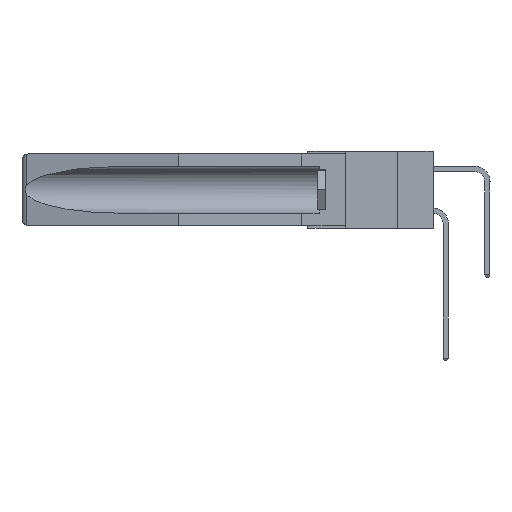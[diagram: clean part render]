
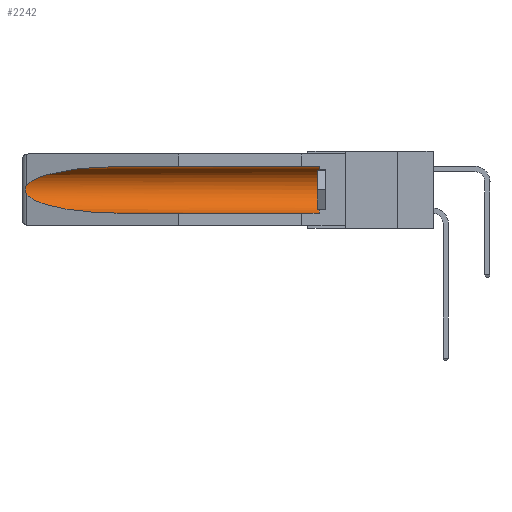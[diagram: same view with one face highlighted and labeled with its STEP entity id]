
A CAD part, left-side view. The second image highlights one B-rep face of the part: STEP entity #2242.
In plain terms, the highlighted cylindrical face has radius 2.857 mm (diameter 5.715 mm), a partial arc.
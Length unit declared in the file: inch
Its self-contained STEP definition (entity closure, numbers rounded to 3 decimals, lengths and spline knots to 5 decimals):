
#13 = VERTEX_POINT ( 'NONE', #9260 ) ;
#589 = ORIENTED_EDGE ( 'NONE', *, *, #10933, .T. ) ;
#742 = CARTESIAN_POINT ( 'NONE',  ( 0.155, 1.07973, -0.059 ) ) ;
#765 = ORIENTED_EDGE ( 'NONE', *, *, #4524, .T. ) ;
#1241 = EDGE_LOOP ( 'NONE', ( #765, #589, #7309, #15230, #18197, #17790 ) ) ;
#1487 = CARTESIAN_POINT ( 'NONE',  ( 0.2675, 1.53308, -0.16763 ) ) ;
#2242 = ADVANCED_FACE ( 'NONE', ( #5202 ), #18464, .F. ) ;
#2340 = DIRECTION ( 'NONE',  ( 0., 0., 1. ) ) ;
#2880 = EDGE_CURVE ( 'NONE', #13, #15522, #5535, .T. ) ;
#3206 = CARTESIAN_POINT ( 'NONE',  ( 0.155, -0.30754, -0.1715 ) ) ;
#3468 = CARTESIAN_POINT ( 'NONE',  ( 0.26537, 1.52718, -0.14972 ) ) ;
#3616 =( BOUNDED_CURVE ( )  B_SPLINE_CURVE ( 3, ( #16390, #7421, #14693, #18410 ),
 .UNSPECIFIED., .F., .F. ) 
 B_SPLINE_CURVE_WITH_KNOTS ( ( 4, 4 ),
 ( 0.1948, 1.5708 ),
 .UNSPECIFIED. ) 
 CURVE ( )  GEOMETRIC_REPRESENTATION_ITEM ( )  RATIONAL_B_SPLINE_CURVE ( ( 1., 0.848, 0.848, 1. ) ) 
 REPRESENTATION_ITEM ( '' )  );
#3846 = EDGE_CURVE ( 'NONE', #11612, #7473, #5758, .T. ) ;
#4273 = DIRECTION ( 'NONE',  ( 0., 1., 0. ) ) ;
#4432 = CARTESIAN_POINT ( 'NONE',  ( 0.155, -0.30754, -0.059 ) ) ;
#4524 = EDGE_CURVE ( 'NONE', #15522, #22439, #20083, .T. ) ;
#5050 = CARTESIAN_POINT ( 'NONE',  ( 0.26597, 1.52961, -0.15275 ) ) ;
#5202 = FACE_OUTER_BOUND ( 'NONE', #1241, .T. ) ;
#5276 = CARTESIAN_POINT ( 'NONE',  ( 0.2675, 1.53308, -0.17534 ) ) ;
#5384 = DIRECTION ( 'NONE',  ( 0., 0., 1. ) ) ;
#5535 = LINE ( 'NONE', #4432, #21639 ) ;
#5715 = CARTESIAN_POINT ( 'NONE',  ( 0.155, -0.30754, -0.284 ) ) ;
#5758 = LINE ( 'NONE', #5715, #20157 ) ;
#7075 = CARTESIAN_POINT ( 'NONE',  ( 0.26537, 1.52718, -0.19328 ) ) ;
#7309 = ORIENTED_EDGE ( 'NONE', *, *, #11479, .T. ) ;
#7373 = CARTESIAN_POINT ( 'NONE',  ( 0.26537, 1.52718, -0.19328 ) ) ;
#7421 = CARTESIAN_POINT ( 'NONE',  ( 0.25451, 1.48313, -0.24835 ) ) ;
#7473 = VERTEX_POINT ( 'NONE', #18750 ) ;
#8163 = EDGE_CURVE ( 'NONE', #11612, #13, #21023, .T. ) ;
#9057 = CARTESIAN_POINT ( 'NONE',  ( 0.25451, 1.48313, -0.09465 ) ) ;
#9208 = CARTESIAN_POINT ( 'NONE',  ( 0.21114, 1.30732, -0.059 ) ) ;
#9260 = CARTESIAN_POINT ( 'NONE',  ( 0.155, 0.126, -0.059 ) ) ;
#9945 = AXIS2_PLACEMENT_3D ( 'NONE', #20248, #14707, #2340 ) ;
#10933 = EDGE_CURVE ( 'NONE', #22439, #11019, #15461, .T. ) ;
#11019 = VERTEX_POINT ( 'NONE', #7373 ) ;
#11479 = EDGE_CURVE ( 'NONE', #11019, #7473, #3616, .T. ) ;
#11612 = VERTEX_POINT ( 'NONE', #22201 ) ;
#14693 = CARTESIAN_POINT ( 'NONE',  ( 0.21114, 1.30732, -0.284 ) ) ;
#14697 = CARTESIAN_POINT ( 'NONE',  ( 0.26537, 1.52718, -0.14972 ) ) ;
#14707 = DIRECTION ( 'NONE',  ( 0., -1., 0. ) ) ;
#15230 = ORIENTED_EDGE ( 'NONE', *, *, #3846, .F. ) ;
#15461 = B_SPLINE_CURVE_WITH_KNOTS ( 'NONE', 3,
 ( #3468, #5050, #16129, #16104, #1487, #5276, #17973, #17895, #19723, #7075 ),
 .UNSPECIFIED., .F., .F.,
 ( 4, 2, 2, 2, 4 ),
 ( 0., 0.00029, 0.00058, 0.00087, 0.00117 ),
 .UNSPECIFIED. ) ;
#15522 = VERTEX_POINT ( 'NONE', #742 ) ;
#16104 = CARTESIAN_POINT ( 'NONE',  ( 0.2673, 1.5327, -0.16383 ) ) ;
#16129 = CARTESIAN_POINT ( 'NONE',  ( 0.26654, 1.53092, -0.15636 ) ) ;
#16315 = DIRECTION ( 'NONE',  ( 0., 1., 0. ) ) ;
#16390 = CARTESIAN_POINT ( 'NONE',  ( 0.26537, 1.52718, -0.19328 ) ) ;
#17627 = CARTESIAN_POINT ( 'NONE',  ( 0.26537, 1.52718, -0.14972 ) ) ;
#17790 = ORIENTED_EDGE ( 'NONE', *, *, #2880, .T. ) ;
#17895 = CARTESIAN_POINT ( 'NONE',  ( 0.26655, 1.53094, -0.18657 ) ) ;
#17973 = CARTESIAN_POINT ( 'NONE',  ( 0.2673, 1.53269, -0.17917 ) ) ;
#18197 = ORIENTED_EDGE ( 'NONE', *, *, #8163, .T. ) ;
#18261 = CARTESIAN_POINT ( 'NONE',  ( 0.155, 1.07973, -0.059 ) ) ;
#18410 = CARTESIAN_POINT ( 'NONE',  ( 0.155, 1.07973, -0.284 ) ) ;
#18411 = DIRECTION ( 'NONE',  ( 0., 1., 0. ) ) ;
#18464 = CYLINDRICAL_SURFACE ( 'NONE', #19734, 0.1125 ) ;
#18750 = CARTESIAN_POINT ( 'NONE',  ( 0.155, 1.07973, -0.284 ) ) ;
#19723 = CARTESIAN_POINT ( 'NONE',  ( 0.26597, 1.5296, -0.19026 ) ) ;
#19734 = AXIS2_PLACEMENT_3D ( 'NONE', #3206, #16315, #5384 ) ;
#20083 =( BOUNDED_CURVE ( )  B_SPLINE_CURVE ( 3, ( #18261, #9208, #9057, #14697 ),
 .UNSPECIFIED., .F., .F. ) 
 B_SPLINE_CURVE_WITH_KNOTS ( ( 4, 4 ),
 ( 4.71239, 6.08839 ),
 .UNSPECIFIED. ) 
 CURVE ( )  GEOMETRIC_REPRESENTATION_ITEM ( )  RATIONAL_B_SPLINE_CURVE ( ( 1., 0.848, 0.848, 1. ) ) 
 REPRESENTATION_ITEM ( '' )  );
#20157 = VECTOR ( 'NONE', #18411, 39.37008 ) ;
#20248 = CARTESIAN_POINT ( 'NONE',  ( 0.155, 0.126, -0.1715 ) ) ;
#21023 = CIRCLE ( 'NONE', #9945, 0.1125 ) ;
#21639 = VECTOR ( 'NONE', #4273, 39.37008 ) ;
#22201 = CARTESIAN_POINT ( 'NONE',  ( 0.155, 0.126, -0.284 ) ) ;
#22439 = VERTEX_POINT ( 'NONE', #17627 ) ;
